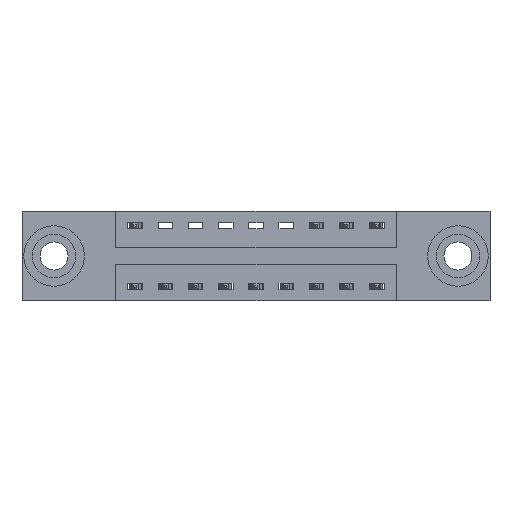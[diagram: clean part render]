
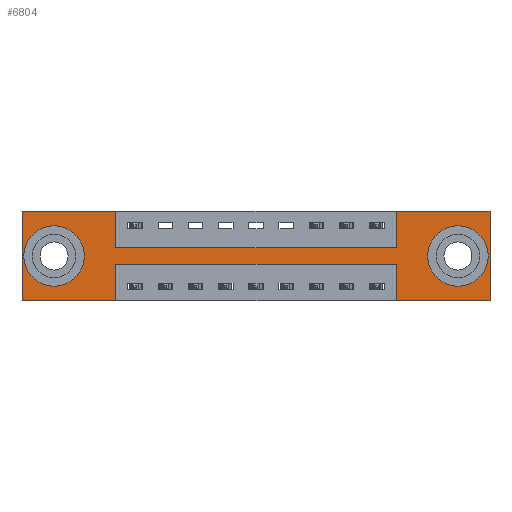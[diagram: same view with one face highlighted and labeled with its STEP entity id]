
A CAD part, front view. The second image highlights one B-rep face of the part: STEP entity #6804.
In plain terms, the highlighted planar face has unit normal (0, -1, 0).
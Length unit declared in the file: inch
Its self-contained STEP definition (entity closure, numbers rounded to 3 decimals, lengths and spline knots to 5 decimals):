
#7 = EDGE_CURVE ( 'NONE', #3268, #8115, #4062, .T. ) ;
#75 = VERTEX_POINT ( 'NONE', #3678 ) ;
#147 = CIRCLE ( 'NONE', #8125, 0.078 ) ;
#227 = LINE ( 'NONE', #4957, #2243 ) ;
#235 = DIRECTION ( 'NONE',  ( 0., 0., -1. ) ) ;
#256 = CARTESIAN_POINT ( 'NONE',  ( 0., 0., 0. ) ) ;
#342 = CARTESIAN_POINT ( 'NONE',  ( 1.8025, 0., -0.185 ) ) ;
#633 = VERTEX_POINT ( 'NONE', #9840 ) ;
#682 = DIRECTION ( 'NONE',  ( -1., 0., 0. ) ) ;
#1034 = CIRCLE ( 'NONE', #3614, 0.078 ) ;
#1053 = PLANE ( 'NONE',  #7449 ) ;
#1096 = CARTESIAN_POINT ( 'NONE',  ( 0.1325, 0., -0.185 ) ) ;
#1098 = VECTOR ( 'NONE', #1194, 39.37008 ) ;
#1103 = AXIS2_PLACEMENT_3D ( 'NONE', #1096, #7018, #1963 ) ;
#1194 = DIRECTION ( 'NONE',  ( -1., 0., 0. ) ) ;
#1203 = DIRECTION ( 'NONE',  ( 0., 0., -1. ) ) ;
#1261 = CARTESIAN_POINT ( 'NONE',  ( 1.5475, 0., 0. ) ) ;
#1382 = LINE ( 'NONE', #9553, #1098 ) ;
#1468 = LINE ( 'NONE', #5394, #5989 ) ;
#1482 = CARTESIAN_POINT ( 'NONE',  ( 0.3875, 0., 0. ) ) ;
#1538 = EDGE_CURVE ( 'NONE', #4209, #2988, #2687, .T. ) ;
#1597 = VERTEX_POINT ( 'NONE', #2723 ) ;
#1642 = CIRCLE ( 'NONE', #7231, 0.078 ) ;
#1798 = EDGE_CURVE ( 'NONE', #5669, #4209, #6790, .T. ) ;
#1819 = CARTESIAN_POINT ( 'NONE',  ( 1.5475, 0., -0.37 ) ) ;
#1963 = DIRECTION ( 'NONE',  ( 0., 0., 1. ) ) ;
#2243 = VECTOR ( 'NONE', #682, 39.37008 ) ;
#2439 = CARTESIAN_POINT ( 'NONE',  ( 1.5475, 0., -0.37 ) ) ;
#2636 = DIRECTION ( 'NONE',  ( 0., 1., 0. ) ) ;
#2687 = LINE ( 'NONE', #3914, #6917 ) ;
#2723 = CARTESIAN_POINT ( 'NONE',  ( 1.935, 0., -0.37 ) ) ;
#2833 = VERTEX_POINT ( 'NONE', #3845 ) ;
#2905 = DIRECTION ( 'NONE',  ( 0., 1., 0. ) ) ;
#2988 = VERTEX_POINT ( 'NONE', #1482 ) ;
#3211 = ORIENTED_EDGE ( 'NONE', *, *, #4086, .T. ) ;
#3268 = VERTEX_POINT ( 'NONE', #6072 ) ;
#3314 = CARTESIAN_POINT ( 'NONE',  ( 0.3875, 0., -0.15 ) ) ;
#3321 = DIRECTION ( 'NONE',  ( 0., 0., 1. ) ) ;
#3338 = VECTOR ( 'NONE', #9722, 39.37008 ) ;
#3362 = ORIENTED_EDGE ( 'NONE', *, *, #10102, .T. ) ;
#3605 = VERTEX_POINT ( 'NONE', #7292 ) ;
#3614 = AXIS2_PLACEMENT_3D ( 'NONE', #342, #6289, #1203 ) ;
#3661 = CARTESIAN_POINT ( 'NONE',  ( 0., 0., -0.37 ) ) ;
#3678 = CARTESIAN_POINT ( 'NONE',  ( 1.5475, 0., -0.15 ) ) ;
#3753 = FACE_BOUND ( 'NONE', #6612, .T. ) ;
#3811 = VECTOR ( 'NONE', #5912, 39.37008 ) ;
#3845 = CARTESIAN_POINT ( 'NONE',  ( 1.8025, 0., -0.263 ) ) ;
#3914 = CARTESIAN_POINT ( 'NONE',  ( 0., 0., 0. ) ) ;
#3927 = DIRECTION ( 'NONE',  ( 1., 0., 0. ) ) ;
#3962 = ORIENTED_EDGE ( 'NONE', *, *, #7525, .T. ) ;
#3964 = EDGE_LOOP ( 'NONE', ( #3989, #3962 ) ) ;
#3989 = ORIENTED_EDGE ( 'NONE', *, *, #4404, .T. ) ;
#4004 = VERTEX_POINT ( 'NONE', #4520 ) ;
#4062 = LINE ( 'NONE', #9482, #3811 ) ;
#4086 = EDGE_CURVE ( 'NONE', #3605, #633, #1642, .T. ) ;
#4104 = EDGE_CURVE ( 'NONE', #8115, #5669, #1382, .T. ) ;
#4111 = DIRECTION ( 'NONE',  ( 0., 0., 1. ) ) ;
#4209 = VERTEX_POINT ( 'NONE', #6575 ) ;
#4304 = EDGE_CURVE ( 'NONE', #10023, #4004, #8719, .T. ) ;
#4404 = EDGE_CURVE ( 'NONE', #6401, #2833, #147, .T. ) ;
#4467 = EDGE_LOOP ( 'NONE', ( #6445, #4804, #5186, #7387, #7349, #9711, #6457, #6463, #5715, #4490, #6495, #5565 ) ) ;
#4490 = ORIENTED_EDGE ( 'NONE', *, *, #1538, .F. ) ;
#4516 = LINE ( 'NONE', #5824, #8409 ) ;
#4520 = CARTESIAN_POINT ( 'NONE',  ( 1.5475, 0., -0.22 ) ) ;
#4567 = VECTOR ( 'NONE', #4111, 39.37008 ) ;
#4804 = ORIENTED_EDGE ( 'NONE', *, *, #10664, .F. ) ;
#4957 = CARTESIAN_POINT ( 'NONE',  ( 0.3875, 0., -0.22 ) ) ;
#5133 = CARTESIAN_POINT ( 'NONE',  ( 0., 0., 0. ) ) ;
#5186 = ORIENTED_EDGE ( 'NONE', *, *, #4304, .F. ) ;
#5366 = DIRECTION ( 'NONE',  ( 0., -1., 0. ) ) ;
#5394 = CARTESIAN_POINT ( 'NONE',  ( 1.5475, 0., 0. ) ) ;
#5565 = ORIENTED_EDGE ( 'NONE', *, *, #4104, .F. ) ;
#5600 = LINE ( 'NONE', #5626, #3338 ) ;
#5626 = CARTESIAN_POINT ( 'NONE',  ( 0.3875, 0., 0. ) ) ;
#5644 = VERTEX_POINT ( 'NONE', #6248 ) ;
#5669 = VERTEX_POINT ( 'NONE', #6285 ) ;
#5715 = ORIENTED_EDGE ( 'NONE', *, *, #9668, .F. ) ;
#5824 = CARTESIAN_POINT ( 'NONE',  ( 0., 0., -0.37 ) ) ;
#5912 = DIRECTION ( 'NONE',  ( 0., 0., -1. ) ) ;
#5984 = VECTOR ( 'NONE', #6678, 39.37008 ) ;
#5989 = VECTOR ( 'NONE', #9465, 39.37008 ) ;
#6072 = CARTESIAN_POINT ( 'NONE',  ( 0.3875, 0., -0.22 ) ) ;
#6106 = CIRCLE ( 'NONE', #1103, 0.078 ) ;
#6240 = LINE ( 'NONE', #3314, #5984 ) ;
#6248 = CARTESIAN_POINT ( 'NONE',  ( 0.3875, 0., -0.15 ) ) ;
#6251 = VERTEX_POINT ( 'NONE', #1261 ) ;
#6285 = CARTESIAN_POINT ( 'NONE',  ( 0., 0., -0.37 ) ) ;
#6289 = DIRECTION ( 'NONE',  ( 0., 1., 0. ) ) ;
#6401 = VERTEX_POINT ( 'NONE', #10613 ) ;
#6445 = ORIENTED_EDGE ( 'NONE', *, *, #7, .F. ) ;
#6457 = ORIENTED_EDGE ( 'NONE', *, *, #6820, .F. ) ;
#6463 = ORIENTED_EDGE ( 'NONE', *, *, #9853, .F. ) ;
#6495 = ORIENTED_EDGE ( 'NONE', *, *, #1798, .F. ) ;
#6575 = CARTESIAN_POINT ( 'NONE',  ( 0., 0., 0. ) ) ;
#6612 = EDGE_LOOP ( 'NONE', ( #3211, #3362 ) ) ;
#6678 = DIRECTION ( 'NONE',  ( 1., 0., 0. ) ) ;
#6790 = LINE ( 'NONE', #256, #4567 ) ;
#6804 = ADVANCED_FACE ( 'NONE', ( #8432, #3753, #8167 ), #1053, .T. ) ;
#6820 = EDGE_CURVE ( 'NONE', #75, #6251, #1468, .T. ) ;
#6917 = VECTOR ( 'NONE', #3927, 39.37008 ) ;
#7018 = DIRECTION ( 'NONE',  ( 0., 1., 0. ) ) ;
#7231 = AXIS2_PLACEMENT_3D ( 'NONE', #7935, #2905, #8743 ) ;
#7292 = CARTESIAN_POINT ( 'NONE',  ( 0.1325, 0., -0.107 ) ) ;
#7349 = ORIENTED_EDGE ( 'NONE', *, *, #9800, .F. ) ;
#7387 = ORIENTED_EDGE ( 'NONE', *, *, #10704, .F. ) ;
#7418 = CARTESIAN_POINT ( 'NONE',  ( 1.935, 0., 0. ) ) ;
#7449 = AXIS2_PLACEMENT_3D ( 'NONE', #3661, #5366, #235 ) ;
#7525 = EDGE_CURVE ( 'NONE', #2833, #6401, #1034, .T. ) ;
#7677 = CARTESIAN_POINT ( 'NONE',  ( 1.8025, 0., -0.185 ) ) ;
#7935 = CARTESIAN_POINT ( 'NONE',  ( 0.1325, 0., -0.185 ) ) ;
#8115 = VERTEX_POINT ( 'NONE', #9216 ) ;
#8125 = AXIS2_PLACEMENT_3D ( 'NONE', #7677, #2636, #8488 ) ;
#8167 = FACE_OUTER_BOUND ( 'NONE', #4467, .T. ) ;
#8271 = DIRECTION ( 'NONE',  ( 0., 0., -1. ) ) ;
#8317 = VECTOR ( 'NONE', #8441, 39.37008 ) ;
#8409 = VECTOR ( 'NONE', #10707, 39.37008 ) ;
#8432 = FACE_BOUND ( 'NONE', #3964, .T. ) ;
#8441 = DIRECTION ( 'NONE',  ( 1., 0., 0. ) ) ;
#8463 = VECTOR ( 'NONE', #3321, 39.37008 ) ;
#8488 = DIRECTION ( 'NONE',  ( 0., 0., -1. ) ) ;
#8672 = VECTOR ( 'NONE', #8271, 39.37008 ) ;
#8719 = LINE ( 'NONE', #2439, #8463 ) ;
#8743 = DIRECTION ( 'NONE',  ( 0., 0., 1. ) ) ;
#8762 = EDGE_CURVE ( 'NONE', #6251, #9739, #10481, .T. ) ;
#9017 = CARTESIAN_POINT ( 'NONE',  ( 1.935, 0., 0. ) ) ;
#9216 = CARTESIAN_POINT ( 'NONE',  ( 0.3875, 0., -0.37 ) ) ;
#9465 = DIRECTION ( 'NONE',  ( 0., 0., 1. ) ) ;
#9482 = CARTESIAN_POINT ( 'NONE',  ( 0.3875, 0., -0.37 ) ) ;
#9553 = CARTESIAN_POINT ( 'NONE',  ( 0., 0., -0.37 ) ) ;
#9668 = EDGE_CURVE ( 'NONE', #2988, #5644, #5600, .T. ) ;
#9711 = ORIENTED_EDGE ( 'NONE', *, *, #8762, .F. ) ;
#9722 = DIRECTION ( 'NONE',  ( 0., 0., -1. ) ) ;
#9739 = VERTEX_POINT ( 'NONE', #9017 ) ;
#9800 = EDGE_CURVE ( 'NONE', #9739, #1597, #10827, .T. ) ;
#9840 = CARTESIAN_POINT ( 'NONE',  ( 0.1325, 0., -0.263 ) ) ;
#9853 = EDGE_CURVE ( 'NONE', #5644, #75, #6240, .T. ) ;
#10023 = VERTEX_POINT ( 'NONE', #1819 ) ;
#10102 = EDGE_CURVE ( 'NONE', #633, #3605, #6106, .T. ) ;
#10481 = LINE ( 'NONE', #5133, #8317 ) ;
#10613 = CARTESIAN_POINT ( 'NONE',  ( 1.8025, 0., -0.107 ) ) ;
#10664 = EDGE_CURVE ( 'NONE', #4004, #3268, #227, .T. ) ;
#10704 = EDGE_CURVE ( 'NONE', #1597, #10023, #4516, .T. ) ;
#10707 = DIRECTION ( 'NONE',  ( -1., 0., 0. ) ) ;
#10827 = LINE ( 'NONE', #7418, #8672 ) ;
